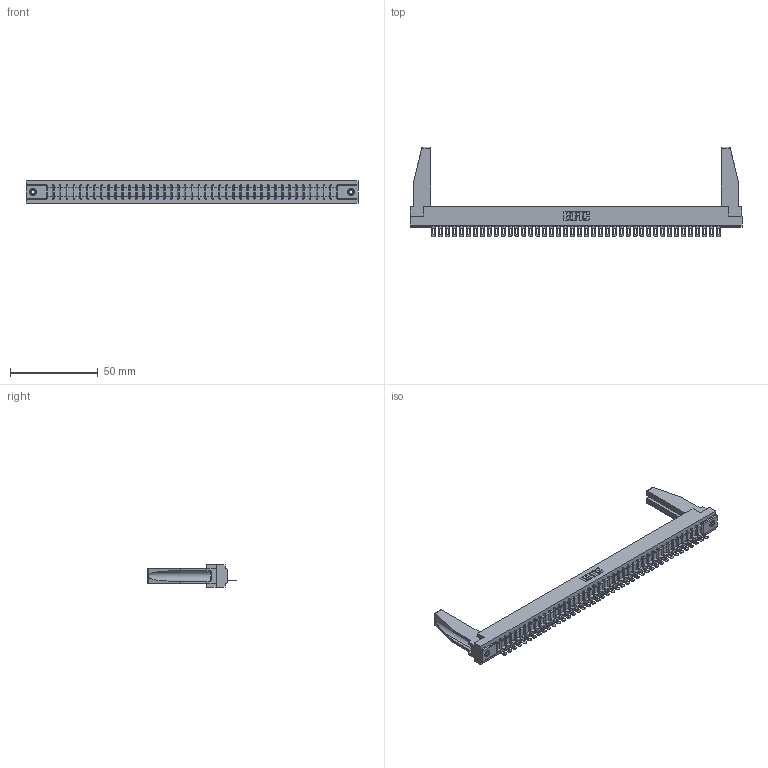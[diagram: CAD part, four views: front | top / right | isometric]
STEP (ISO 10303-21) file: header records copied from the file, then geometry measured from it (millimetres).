
FILE_DESCRIPTION (( 'STEP AP203' ), '1' );
FILE_NAME ('307-042-501-178.STEP', '2019-09-05T11:38:31', ( '' ), ( '' ), 'SwSTEP 2.0', 'SolidWorks 2016', '' );
FILE_SCHEMA (( 'CONFIG_CONTROL_DESIGN' ));
Length unit declared in the file: inch
Products named in the file (5): 307-220-078; 307-290-002_501; 307 Part_.156 Dia Mounting Holes; 345-250-001_345-250-001-102; 307-042-501-178
Assembly tree (47 placements, depth 2):
  307-042-501-178
    307 Part_.156 Dia Mounting Holes
    307-290-002_501  x42
    307-220-078  x2
    345-250-001_345-250-001-102  x2
Bounding box: 189.43 x 51.13 x 12.7 mm (x, y, z)
Volume: 24301.7 mm3; surface area: 29643.8 mm2
Topology: 47 solids, 47 shells, 3483 faces, 10649 edges, 6974 vertices
Faces by surface type: plane 2002, cylinder 1379, sphere 86, cone 12, torus 4
Entity records: 39239 total; most frequent: CARTESIAN_POINT 6618, ORIENTED_EDGE 6564, DIRECTION 6390, EDGE_CURVE 3282, LINE 2514, VECTOR 2514, VERTEX_POINT 2124, AXIS2_PLACEMENT_3D 1938
